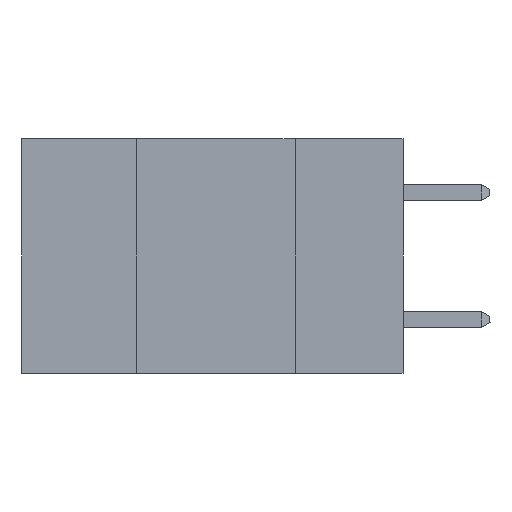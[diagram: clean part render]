
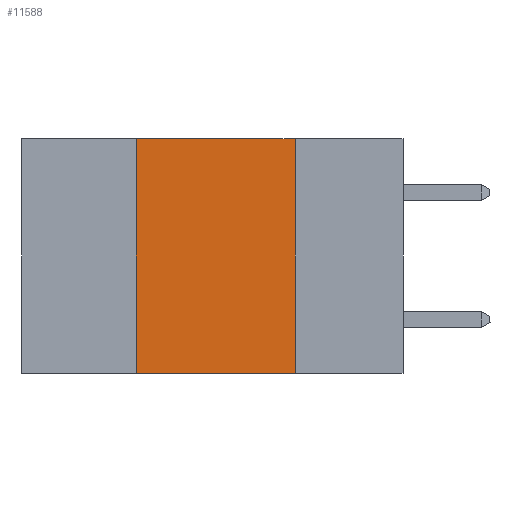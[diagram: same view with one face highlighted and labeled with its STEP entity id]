
A CAD part, left-side view. The second image highlights one B-rep face of the part: STEP entity #11588.
In plain terms, the highlighted planar face has unit normal (-1, 0, 0).
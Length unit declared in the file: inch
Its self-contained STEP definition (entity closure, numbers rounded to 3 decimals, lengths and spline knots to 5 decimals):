
#53 = VECTOR ( 'NONE', #17424, 39.37008 ) ;
#184 = VERTEX_POINT ( 'NONE', #21196 ) ;
#226 = LINE ( 'NONE', #19172, #53 ) ;
#1608 = DIRECTION ( 'NONE',  ( 0., 0., -1. ) ) ;
#3605 = DIRECTION ( 'NONE',  ( 0., -1., 0. ) ) ;
#4383 = ORIENTED_EDGE ( 'NONE', *, *, #24166, .F. ) ;
#5618 = VERTEX_POINT ( 'NONE', #11499 ) ;
#7266 = VECTOR ( 'NONE', #20023, 39.37008 ) ;
#8995 = DIRECTION ( 'NONE',  ( 0., 0., 1. ) ) ;
#9497 = DIRECTION ( 'NONE',  ( 1., 0., 0. ) ) ;
#10432 = EDGE_CURVE ( 'NONE', #23685, #15474, #226, .T. ) ;
#10994 = PLANE ( 'NONE',  #16799 ) ;
#11499 = CARTESIAN_POINT ( 'NONE',  ( 0., 0.42, 0. ) ) ;
#11588 = ADVANCED_FACE ( 'NONE', ( #12847 ), #10994, .F. ) ;
#11939 = EDGE_CURVE ( 'NONE', #184, #15474, #16202, .T. ) ;
#12847 = FACE_OUTER_BOUND ( 'NONE', #22397, .T. ) ;
#14571 = CARTESIAN_POINT ( 'NONE',  ( 0., 0.17, -0.37 ) ) ;
#15474 = VERTEX_POINT ( 'NONE', #14571 ) ;
#15828 = ORIENTED_EDGE ( 'NONE', *, *, #11939, .T. ) ;
#16202 = LINE ( 'NONE', #18181, #7266 ) ;
#16799 = AXIS2_PLACEMENT_3D ( 'NONE', #20419, #9497, #1608 ) ;
#17424 = DIRECTION ( 'NONE',  ( 0., 0., -1. ) ) ;
#18181 = CARTESIAN_POINT ( 'NONE',  ( 0., 0.6, -0.37 ) ) ;
#19172 = CARTESIAN_POINT ( 'NONE',  ( 0., 0.17, 0. ) ) ;
#19819 = CARTESIAN_POINT ( 'NONE',  ( 0., 0.17, 0. ) ) ;
#20023 = DIRECTION ( 'NONE',  ( 0., -1., 0. ) ) ;
#20419 = CARTESIAN_POINT ( 'NONE',  ( 0., 0.6, 0. ) ) ;
#20458 = VECTOR ( 'NONE', #8995, 39.37008 ) ;
#20518 = CARTESIAN_POINT ( 'NONE',  ( 0., 0.42, 0. ) ) ;
#20779 = VECTOR ( 'NONE', #3605, 39.37008 ) ;
#21196 = CARTESIAN_POINT ( 'NONE',  ( 0., 0.42, -0.37 ) ) ;
#22102 = ORIENTED_EDGE ( 'NONE', *, *, #22479, .F. ) ;
#22397 = EDGE_LOOP ( 'NONE', ( #24393, #22102, #4383, #15828 ) ) ;
#22479 = EDGE_CURVE ( 'NONE', #5618, #23685, #24041, .T. ) ;
#22534 = CARTESIAN_POINT ( 'NONE',  ( 0., 0.6, 0. ) ) ;
#23685 = VERTEX_POINT ( 'NONE', #19819 ) ;
#24041 = LINE ( 'NONE', #22534, #20779 ) ;
#24106 = LINE ( 'NONE', #20518, #20458 ) ;
#24166 = EDGE_CURVE ( 'NONE', #184, #5618, #24106, .T. ) ;
#24393 = ORIENTED_EDGE ( 'NONE', *, *, #10432, .F. ) ;
